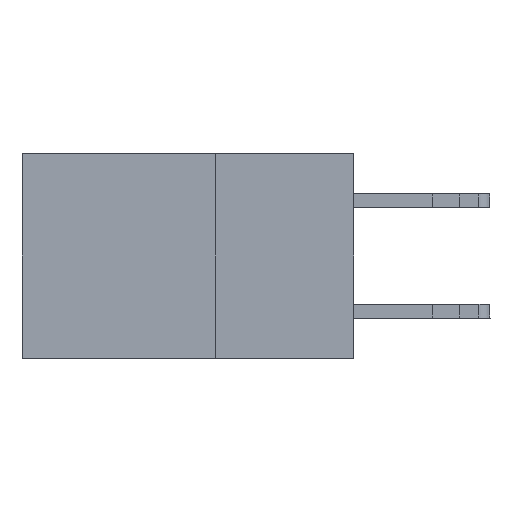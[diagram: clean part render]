
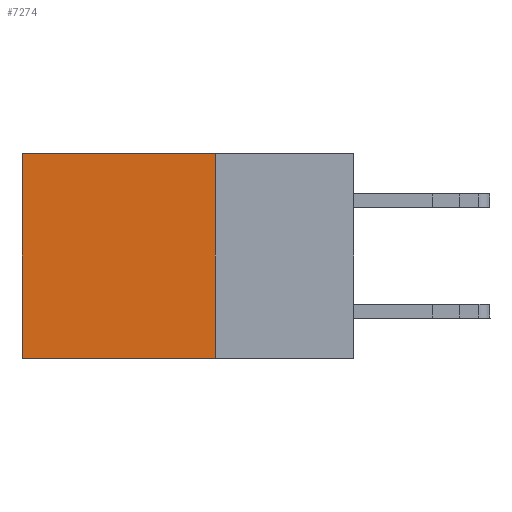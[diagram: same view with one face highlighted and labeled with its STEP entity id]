
A CAD part, left-side view. The second image highlights one B-rep face of the part: STEP entity #7274.
In plain terms, the highlighted planar face has unit normal (-1, 0, 0).
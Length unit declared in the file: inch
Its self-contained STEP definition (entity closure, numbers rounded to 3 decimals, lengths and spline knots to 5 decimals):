
#1681 = DIRECTION ( 'NONE',  ( 1., 0., 0. ) ) ;
#1889 = DIRECTION ( 'NONE',  ( 0., 0., -1. ) ) ;
#2650 = CARTESIAN_POINT ( 'NONE',  ( 0.2875, 0.25, -0.37 ) ) ;
#2773 = CARTESIAN_POINT ( 'NONE',  ( 0.2875, 0.25, 0. ) ) ;
#3083 = ORIENTED_EDGE ( 'NONE', *, *, #5173, .T. ) ;
#5173 = EDGE_CURVE ( 'NONE', #7865, #6786, #9521, .T. ) ;
#5685 = VECTOR ( 'NONE', #1889, 39.37008 ) ;
#6287 = VERTEX_POINT ( 'NONE', #14011 ) ;
#6786 = VERTEX_POINT ( 'NONE', #20910 ) ;
#7274 = ADVANCED_FACE ( 'NONE', ( #12651 ), #22170, .F. ) ;
#7865 = VERTEX_POINT ( 'NONE', #20876 ) ;
#8786 = LINE ( 'NONE', #23622, #9816 ) ;
#9521 = LINE ( 'NONE', #13445, #5685 ) ;
#9777 = VECTOR ( 'NONE', #17178, 39.37008 ) ;
#9816 = VECTOR ( 'NONE', #14203, 39.37008 ) ;
#9918 = LINE ( 'NONE', #22777, #9777 ) ;
#12067 = ORIENTED_EDGE ( 'NONE', *, *, #23668, .F. ) ;
#12651 = FACE_OUTER_BOUND ( 'NONE', #21108, .T. ) ;
#13089 = ORIENTED_EDGE ( 'NONE', *, *, #21650, .F. ) ;
#13445 = CARTESIAN_POINT ( 'NONE',  ( 0.2875, 0.6, 0. ) ) ;
#14011 = CARTESIAN_POINT ( 'NONE',  ( 0.2875, 0.25, 0. ) ) ;
#14074 = DIRECTION ( 'NONE',  ( 0., 1., 0. ) ) ;
#14203 = DIRECTION ( 'NONE',  ( 0., 0., -1. ) ) ;
#15487 = ORIENTED_EDGE ( 'NONE', *, *, #21058, .T. ) ;
#16440 = DIRECTION ( 'NONE',  ( 0., 0., -1. ) ) ;
#16792 = AXIS2_PLACEMENT_3D ( 'NONE', #18684, #1681, #16440 ) ;
#17178 = DIRECTION ( 'NONE',  ( 0., 1., 0. ) ) ;
#18684 = CARTESIAN_POINT ( 'NONE',  ( 0.2875, 0.25, 0. ) ) ;
#19660 = LINE ( 'NONE', #2773, #20665 ) ;
#20665 = VECTOR ( 'NONE', #14074, 39.37008 ) ;
#20876 = CARTESIAN_POINT ( 'NONE',  ( 0.2875, 0.6, 0. ) ) ;
#20910 = CARTESIAN_POINT ( 'NONE',  ( 0.2875, 0.6, -0.37 ) ) ;
#21045 = VERTEX_POINT ( 'NONE', #2650 ) ;
#21058 = EDGE_CURVE ( 'NONE', #6287, #7865, #19660, .T. ) ;
#21108 = EDGE_LOOP ( 'NONE', ( #3083, #13089, #12067, #15487 ) ) ;
#21650 = EDGE_CURVE ( 'NONE', #21045, #6786, #9918, .T. ) ;
#22170 = PLANE ( 'NONE',  #16792 ) ;
#22777 = CARTESIAN_POINT ( 'NONE',  ( 0.2875, 0.25, -0.37 ) ) ;
#23622 = CARTESIAN_POINT ( 'NONE',  ( 0.2875, 0.25, 0. ) ) ;
#23668 = EDGE_CURVE ( 'NONE', #6287, #21045, #8786, .T. ) ;
